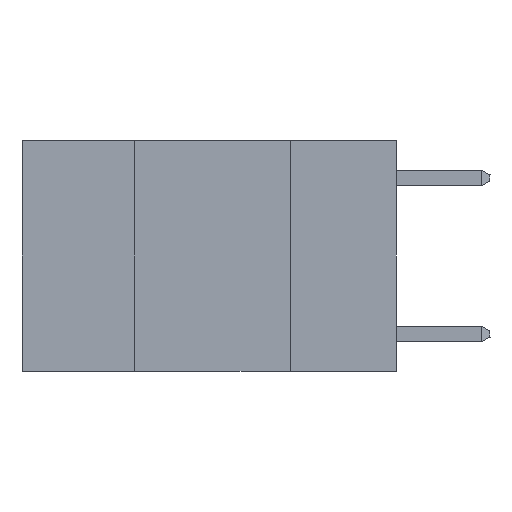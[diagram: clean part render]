
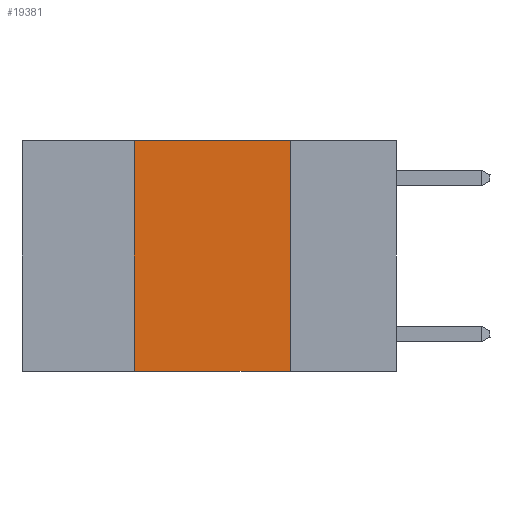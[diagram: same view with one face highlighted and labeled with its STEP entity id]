
A CAD part, left-side view. The second image highlights one B-rep face of the part: STEP entity #19381.
In plain terms, the highlighted planar face has unit normal (-1, 0, 0).
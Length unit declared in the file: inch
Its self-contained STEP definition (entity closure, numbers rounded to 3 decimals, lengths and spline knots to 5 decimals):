
#65 = ORIENTED_EDGE ( 'NONE', *, *, #3048, .F. ) ;
#1162 = DIRECTION ( 'NONE',  ( 0., 0., -1. ) ) ;
#2761 = FACE_OUTER_BOUND ( 'NONE', #4712, .T. ) ;
#3048 = EDGE_CURVE ( 'NONE', #12843, #4004, #22365, .T. ) ;
#4004 = VERTEX_POINT ( 'NONE', #21281 ) ;
#4712 = EDGE_LOOP ( 'NONE', ( #7046, #65, #6531, #24072 ) ) ;
#4862 = CARTESIAN_POINT ( 'NONE',  ( 0., 0.6, -0.37 ) ) ;
#6045 = VECTOR ( 'NONE', #16979, 39.37008 ) ;
#6109 = EDGE_CURVE ( 'NONE', #7049, #12843, #16409, .T. ) ;
#6192 = CARTESIAN_POINT ( 'NONE',  ( 0., 0.42, -0.37 ) ) ;
#6347 = AXIS2_PLACEMENT_3D ( 'NONE', #17601, #12037, #1162 ) ;
#6531 = ORIENTED_EDGE ( 'NONE', *, *, #6109, .F. ) ;
#7046 = ORIENTED_EDGE ( 'NONE', *, *, #9872, .F. ) ;
#7049 = VERTEX_POINT ( 'NONE', #6192 ) ;
#7271 = CARTESIAN_POINT ( 'NONE',  ( 0., 0.42, 0. ) ) ;
#9156 = VECTOR ( 'NONE', #13345, 39.37008 ) ;
#9164 = CARTESIAN_POINT ( 'NONE',  ( 0., 0.17, -0.37 ) ) ;
#9872 = EDGE_CURVE ( 'NONE', #4004, #10358, #13532, .T. ) ;
#10358 = VERTEX_POINT ( 'NONE', #9164 ) ;
#12037 = DIRECTION ( 'NONE',  ( 1., 0., 0. ) ) ;
#12843 = VERTEX_POINT ( 'NONE', #19929 ) ;
#13222 = CARTESIAN_POINT ( 'NONE',  ( 0., 0.6, 0. ) ) ;
#13345 = DIRECTION ( 'NONE',  ( 0., -1., 0. ) ) ;
#13532 = LINE ( 'NONE', #16855, #6045 ) ;
#13903 = PLANE ( 'NONE',  #6347 ) ;
#14424 = EDGE_CURVE ( 'NONE', #7049, #10358, #21908, .T. ) ;
#15984 = DIRECTION ( 'NONE',  ( 0., -1., 0. ) ) ;
#16409 = LINE ( 'NONE', #7271, #21367 ) ;
#16855 = CARTESIAN_POINT ( 'NONE',  ( 0., 0.17, 0. ) ) ;
#16979 = DIRECTION ( 'NONE',  ( 0., 0., -1. ) ) ;
#17601 = CARTESIAN_POINT ( 'NONE',  ( 0., 0.6, 0. ) ) ;
#19381 = ADVANCED_FACE ( 'NONE', ( #2761 ), #13903, .F. ) ;
#19929 = CARTESIAN_POINT ( 'NONE',  ( 0., 0.42, 0. ) ) ;
#21185 = VECTOR ( 'NONE', #15984, 39.37008 ) ;
#21281 = CARTESIAN_POINT ( 'NONE',  ( 0., 0.17, 0. ) ) ;
#21367 = VECTOR ( 'NONE', #24295, 39.37008 ) ;
#21908 = LINE ( 'NONE', #4862, #21185 ) ;
#22365 = LINE ( 'NONE', #13222, #9156 ) ;
#24072 = ORIENTED_EDGE ( 'NONE', *, *, #14424, .T. ) ;
#24295 = DIRECTION ( 'NONE',  ( 0., 0., 1. ) ) ;
